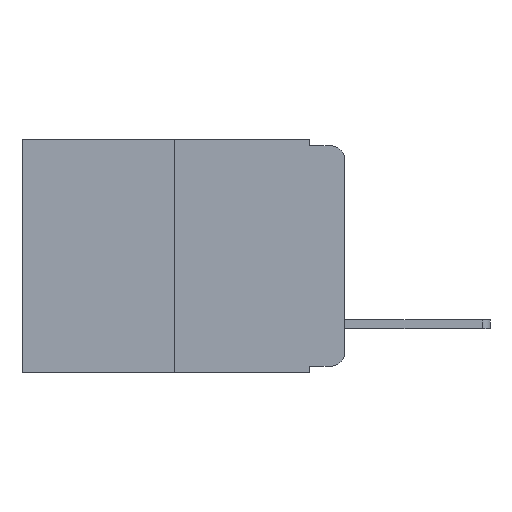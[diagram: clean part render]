
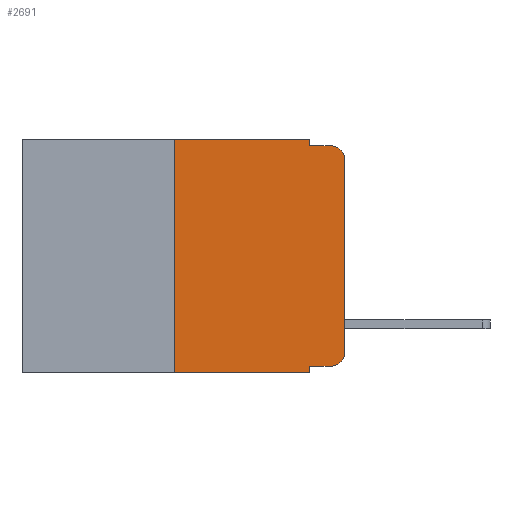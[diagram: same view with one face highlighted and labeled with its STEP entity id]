
A CAD part, left-side view. The second image highlights one B-rep face of the part: STEP entity #2691.
In plain terms, the highlighted planar face has unit normal (-1, 0, 0).
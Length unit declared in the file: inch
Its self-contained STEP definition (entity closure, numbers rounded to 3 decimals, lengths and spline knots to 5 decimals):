
#81 = VECTOR ( 'NONE', #16706, 39.37008 ) ;
#96 = DIRECTION ( 'NONE',  ( 0., -1., 0. ) ) ;
#153 = VECTOR ( 'NONE', #16613, 39.37008 ) ;
#316 = EDGE_CURVE ( 'NONE', #11205, #3663, #4458, .T. ) ;
#414 = CARTESIAN_POINT ( 'NONE',  ( 0., 0.051, -0.01 ) ) ;
#998 = CARTESIAN_POINT ( 'NONE',  ( 0., 0.473, -0.343 ) ) ;
#1472 = VECTOR ( 'NONE', #12009, 39.37008 ) ;
#1587 = VECTOR ( 'NONE', #4571, 39.37008 ) ;
#1612 = VERTEX_POINT ( 'NONE', #3221 ) ;
#1694 = DIRECTION ( 'NONE',  ( -1., 0., 0. ) ) ;
#1707 = CARTESIAN_POINT ( 'NONE',  ( 0., 0.02, -0.313 ) ) ;
#1931 = LINE ( 'NONE', #1938, #8827 ) ;
#1938 = CARTESIAN_POINT ( 'NONE',  ( 0., 0.051, 0. ) ) ;
#2021 = LINE ( 'NONE', #3169, #1587 ) ;
#2121 = FACE_OUTER_BOUND ( 'NONE', #2258, .T. ) ;
#2258 = EDGE_LOOP ( 'NONE', ( #13153, #16572, #13542, #16980, #13946, #17386, #3607, #14362, #11285, #14768 ) ) ;
#2691 = ADVANCED_FACE ( 'NONE', ( #2121 ), #13724, .F. ) ;
#3169 = CARTESIAN_POINT ( 'NONE',  ( 0., 0.473, 0. ) ) ;
#3221 = CARTESIAN_POINT ( 'NONE',  ( 0., 0.051, 0. ) ) ;
#3566 = AXIS2_PLACEMENT_3D ( 'NONE', #1707, #1694, #12188 ) ;
#3607 = ORIENTED_EDGE ( 'NONE', *, *, #5609, .T. ) ;
#3663 = VERTEX_POINT ( 'NONE', #13839 ) ;
#4201 = DIRECTION ( 'NONE',  ( 0., 0., 1. ) ) ;
#4315 = LINE ( 'NONE', #414, #153 ) ;
#4458 = LINE ( 'NONE', #6573, #10130 ) ;
#4571 = DIRECTION ( 'NONE',  ( 0., -1., 0. ) ) ;
#5126 = VERTEX_POINT ( 'NONE', #15541 ) ;
#5175 = CARTESIAN_POINT ( 'NONE',  ( 0., 0.051, -0.333 ) ) ;
#5177 = LINE ( 'NONE', #13355, #1472 ) ;
#5222 = CARTESIAN_POINT ( 'NONE',  ( 0., 0.02, -0.03 ) ) ;
#5383 = EDGE_CURVE ( 'NONE', #6644, #11205, #10322, .T. ) ;
#5609 = EDGE_CURVE ( 'NONE', #8221, #7043, #10100, .T. ) ;
#5675 = VECTOR ( 'NONE', #96, 39.37008 ) ;
#5791 = CARTESIAN_POINT ( 'NONE',  ( 0., 0.051, -0.343 ) ) ;
#6287 = EDGE_CURVE ( 'NONE', #9178, #6644, #9280, .T. ) ;
#6573 = CARTESIAN_POINT ( 'NONE',  ( 0., 0., 0. ) ) ;
#6604 = DIRECTION ( 'NONE',  ( 0., 0., -1. ) ) ;
#6644 = VERTEX_POINT ( 'NONE', #7007 ) ;
#6839 = AXIS2_PLACEMENT_3D ( 'NONE', #5222, #14556, #6604 ) ;
#7007 = CARTESIAN_POINT ( 'NONE',  ( 0., 0.02, -0.333 ) ) ;
#7043 = VERTEX_POINT ( 'NONE', #5791 ) ;
#7224 = EDGE_CURVE ( 'NONE', #9178, #7043, #1931, .T. ) ;
#7459 = CARTESIAN_POINT ( 'NONE',  ( 0., 0., -0.313 ) ) ;
#8111 = EDGE_CURVE ( 'NONE', #8221, #5126, #5177, .T. ) ;
#8221 = VERTEX_POINT ( 'NONE', #16170 ) ;
#8827 = VECTOR ( 'NONE', #14051, 39.37008 ) ;
#9023 = EDGE_CURVE ( 'NONE', #1612, #12037, #11862, .T. ) ;
#9079 = DIRECTION ( 'NONE',  ( 0., -1., 0. ) ) ;
#9178 = VERTEX_POINT ( 'NONE', #5175 ) ;
#9280 = LINE ( 'NONE', #12003, #12402 ) ;
#10100 = LINE ( 'NONE', #998, #5675 ) ;
#10122 = CIRCLE ( 'NONE', #6839, 0.02 ) ;
#10130 = VECTOR ( 'NONE', #4201, 39.37008 ) ;
#10270 = CARTESIAN_POINT ( 'NONE',  ( 0., 0.02, -0.01 ) ) ;
#10322 = CIRCLE ( 'NONE', #3566, 0.02 ) ;
#11195 = AXIS2_PLACEMENT_3D ( 'NONE', #12951, #14665, #12994 ) ;
#11205 = VERTEX_POINT ( 'NONE', #7459 ) ;
#11285 = ORIENTED_EDGE ( 'NONE', *, *, #6287, .T. ) ;
#11862 = LINE ( 'NONE', #15474, #81 ) ;
#12003 = CARTESIAN_POINT ( 'NONE',  ( 0., 0.051, -0.333 ) ) ;
#12009 = DIRECTION ( 'NONE',  ( 0., 0., 1. ) ) ;
#12037 = VERTEX_POINT ( 'NONE', #17235 ) ;
#12188 = DIRECTION ( 'NONE',  ( 0., 0., -1. ) ) ;
#12402 = VECTOR ( 'NONE', #9079, 39.37008 ) ;
#12951 = CARTESIAN_POINT ( 'NONE',  ( 0., 0.473, 0. ) ) ;
#12994 = DIRECTION ( 'NONE',  ( 0., 0., -1. ) ) ;
#13153 = ORIENTED_EDGE ( 'NONE', *, *, #316, .T. ) ;
#13355 = CARTESIAN_POINT ( 'NONE',  ( 0., 0.25, 0. ) ) ;
#13448 = EDGE_CURVE ( 'NONE', #12037, #16304, #4315, .T. ) ;
#13542 = ORIENTED_EDGE ( 'NONE', *, *, #13448, .F. ) ;
#13724 = PLANE ( 'NONE',  #11195 ) ;
#13839 = CARTESIAN_POINT ( 'NONE',  ( 0., 0., -0.03 ) ) ;
#13946 = ORIENTED_EDGE ( 'NONE', *, *, #16163, .F. ) ;
#14051 = DIRECTION ( 'NONE',  ( 0., 0., -1. ) ) ;
#14362 = ORIENTED_EDGE ( 'NONE', *, *, #7224, .F. ) ;
#14556 = DIRECTION ( 'NONE',  ( -1., 0., 0. ) ) ;
#14665 = DIRECTION ( 'NONE',  ( 1., 0., 0. ) ) ;
#14768 = ORIENTED_EDGE ( 'NONE', *, *, #5383, .T. ) ;
#15474 = CARTESIAN_POINT ( 'NONE',  ( 0., 0.051, 0. ) ) ;
#15541 = CARTESIAN_POINT ( 'NONE',  ( 0., 0.25, 0. ) ) ;
#16163 = EDGE_CURVE ( 'NONE', #5126, #1612, #2021, .T. ) ;
#16170 = CARTESIAN_POINT ( 'NONE',  ( 0., 0.25, -0.343 ) ) ;
#16304 = VERTEX_POINT ( 'NONE', #10270 ) ;
#16572 = ORIENTED_EDGE ( 'NONE', *, *, #16902, .T. ) ;
#16613 = DIRECTION ( 'NONE',  ( 0., -1., 0. ) ) ;
#16706 = DIRECTION ( 'NONE',  ( 0., 0., -1. ) ) ;
#16902 = EDGE_CURVE ( 'NONE', #3663, #16304, #10122, .T. ) ;
#16980 = ORIENTED_EDGE ( 'NONE', *, *, #9023, .F. ) ;
#17235 = CARTESIAN_POINT ( 'NONE',  ( 0., 0.051, -0.01 ) ) ;
#17386 = ORIENTED_EDGE ( 'NONE', *, *, #8111, .F. ) ;
